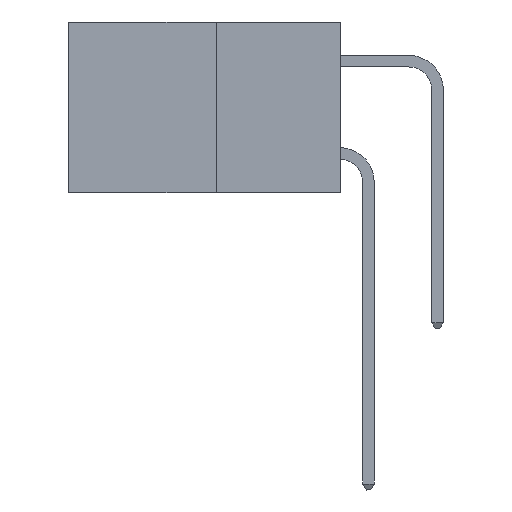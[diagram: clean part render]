
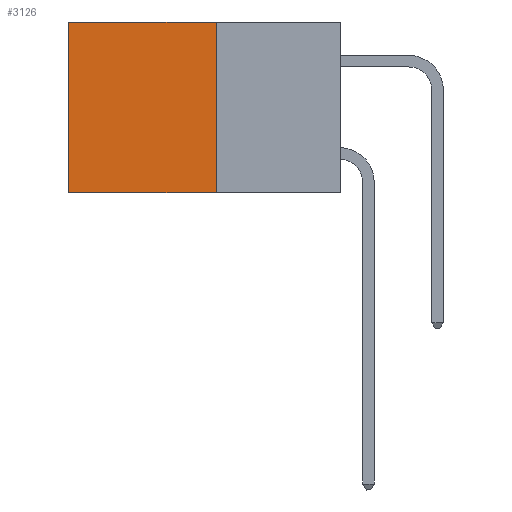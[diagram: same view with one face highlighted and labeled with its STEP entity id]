
A CAD part, left-side view. The second image highlights one B-rep face of the part: STEP entity #3126.
In plain terms, the highlighted planar face has unit normal (-1, 0, 0).
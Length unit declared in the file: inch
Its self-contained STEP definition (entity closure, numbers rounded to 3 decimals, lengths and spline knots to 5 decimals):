
#29 = EDGE_CURVE ( 'NONE', #1840, #589, #6377, .T. ) ;
#414 = FACE_OUTER_BOUND ( 'NONE', #1383, .T. ) ;
#589 = VERTEX_POINT ( 'NONE', #5472 ) ;
#858 = CARTESIAN_POINT ( 'NONE',  ( 0.277, 0.27, -0.37 ) ) ;
#1201 = VECTOR ( 'NONE', #11086, 39.37008 ) ;
#1263 = VERTEX_POINT ( 'NONE', #7157 ) ;
#1383 = EDGE_LOOP ( 'NONE', ( #2348, #12799, #10027, #10875 ) ) ;
#1627 = DIRECTION ( 'NONE',  ( 0., 0., -1. ) ) ;
#1731 = EDGE_CURVE ( 'NONE', #589, #1263, #10953, .T. ) ;
#1782 = DIRECTION ( 'NONE',  ( 0., 1., 0. ) ) ;
#1840 = VERTEX_POINT ( 'NONE', #10624 ) ;
#1976 = VECTOR ( 'NONE', #1627, 39.37008 ) ;
#1979 = DIRECTION ( 'NONE',  ( 0., 0., -1. ) ) ;
#2348 = ORIENTED_EDGE ( 'NONE', *, *, #1731, .T. ) ;
#3004 = AXIS2_PLACEMENT_3D ( 'NONE', #3078, #5249, #1979 ) ;
#3078 = CARTESIAN_POINT ( 'NONE',  ( 0.277, 0.27, -0.37 ) ) ;
#3126 = ADVANCED_FACE ( 'NONE', ( #414 ), #6785, .F. ) ;
#5249 = DIRECTION ( 'NONE',  ( 1., 0., 0. ) ) ;
#5264 = CARTESIAN_POINT ( 'NONE',  ( 0.277, 0.59, -0.37 ) ) ;
#5268 = DIRECTION ( 'NONE',  ( 0., 1., 0. ) ) ;
#5472 = CARTESIAN_POINT ( 'NONE',  ( 0.277, 0.59, 0. ) ) ;
#6377 = LINE ( 'NONE', #8793, #9037 ) ;
#6785 = PLANE ( 'NONE',  #3004 ) ;
#7157 = CARTESIAN_POINT ( 'NONE',  ( 0.277, 0.59, -0.37 ) ) ;
#7217 = LINE ( 'NONE', #9961, #1201 ) ;
#7298 = VERTEX_POINT ( 'NONE', #858 ) ;
#8793 = CARTESIAN_POINT ( 'NONE',  ( 0.277, 0.27, 0. ) ) ;
#9037 = VECTOR ( 'NONE', #1782, 39.37008 ) ;
#9961 = CARTESIAN_POINT ( 'NONE',  ( 0.277, 0.27, -0.37 ) ) ;
#10027 = ORIENTED_EDGE ( 'NONE', *, *, #14258, .F. ) ;
#10266 = LINE ( 'NONE', #13011, #13420 ) ;
#10624 = CARTESIAN_POINT ( 'NONE',  ( 0.277, 0.27, 0. ) ) ;
#10875 = ORIENTED_EDGE ( 'NONE', *, *, #29, .T. ) ;
#10953 = LINE ( 'NONE', #5264, #1976 ) ;
#11086 = DIRECTION ( 'NONE',  ( 0., 0., -1. ) ) ;
#12111 = EDGE_CURVE ( 'NONE', #7298, #1263, #10266, .T. ) ;
#12799 = ORIENTED_EDGE ( 'NONE', *, *, #12111, .F. ) ;
#13011 = CARTESIAN_POINT ( 'NONE',  ( 0.277, 0.27, -0.37 ) ) ;
#13420 = VECTOR ( 'NONE', #5268, 39.37008 ) ;
#14258 = EDGE_CURVE ( 'NONE', #1840, #7298, #7217, .T. ) ;
